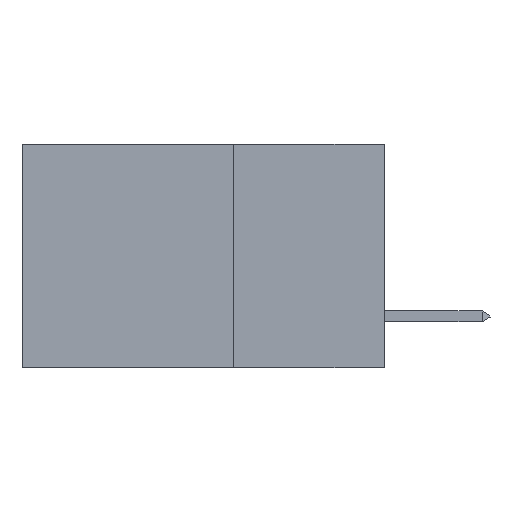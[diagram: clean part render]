
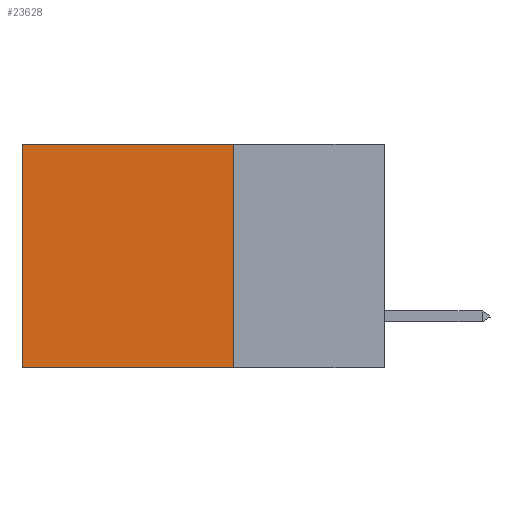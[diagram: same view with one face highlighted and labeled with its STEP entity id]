
A CAD part, left-side view. The second image highlights one B-rep face of the part: STEP entity #23628.
In plain terms, the highlighted planar face has unit normal (-1, 0, 0).
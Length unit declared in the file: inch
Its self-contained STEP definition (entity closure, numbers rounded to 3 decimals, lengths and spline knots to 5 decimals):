
#699 = FACE_OUTER_BOUND ( 'NONE', #1510, .T. ) ;
#1510 = EDGE_LOOP ( 'NONE', ( #21617, #4428, #1871, #13082 ) ) ;
#1652 = VECTOR ( 'NONE', #9317, 39.37008 ) ;
#1871 = ORIENTED_EDGE ( 'NONE', *, *, #20863, .F. ) ;
#3248 = CARTESIAN_POINT ( 'NONE',  ( 0.2875, 0.6, 0. ) ) ;
#3627 = VERTEX_POINT ( 'NONE', #20398 ) ;
#4079 = CARTESIAN_POINT ( 'NONE',  ( 0.2875, 0.25, -0.37 ) ) ;
#4428 = ORIENTED_EDGE ( 'NONE', *, *, #23830, .F. ) ;
#5561 = DIRECTION ( 'NONE',  ( 0., 0., -1. ) ) ;
#5659 = PLANE ( 'NONE',  #22956 ) ;
#5740 = VERTEX_POINT ( 'NONE', #3248 ) ;
#7494 = VECTOR ( 'NONE', #15050, 39.37008 ) ;
#7834 = CARTESIAN_POINT ( 'NONE',  ( 0.2875, 0.6, -0.37 ) ) ;
#8521 = EDGE_CURVE ( 'NONE', #21732, #5740, #12229, .T. ) ;
#8825 = VERTEX_POINT ( 'NONE', #7834 ) ;
#9296 = CARTESIAN_POINT ( 'NONE',  ( 0.2875, 0.25, 0. ) ) ;
#9317 = DIRECTION ( 'NONE',  ( 0., 1., 0. ) ) ;
#10477 = CARTESIAN_POINT ( 'NONE',  ( 0.2875, 0.6, 0. ) ) ;
#11054 = EDGE_CURVE ( 'NONE', #5740, #8825, #20104, .T. ) ;
#12229 = LINE ( 'NONE', #17716, #1652 ) ;
#13082 = ORIENTED_EDGE ( 'NONE', *, *, #8521, .T. ) ;
#15039 = VECTOR ( 'NONE', #23583, 39.37008 ) ;
#15050 = DIRECTION ( 'NONE',  ( 0., 1., 0. ) ) ;
#15095 = DIRECTION ( 'NONE',  ( 0., 0., -1. ) ) ;
#15701 = LINE ( 'NONE', #4079, #7494 ) ;
#15866 = LINE ( 'NONE', #9296, #18580 ) ;
#17716 = CARTESIAN_POINT ( 'NONE',  ( 0.2875, 0.25, 0. ) ) ;
#18580 = VECTOR ( 'NONE', #5561, 39.37008 ) ;
#18710 = DIRECTION ( 'NONE',  ( 1., 0., 0. ) ) ;
#18781 = CARTESIAN_POINT ( 'NONE',  ( 0.2875, 0.25, 0. ) ) ;
#20104 = LINE ( 'NONE', #10477, #15039 ) ;
#20398 = CARTESIAN_POINT ( 'NONE',  ( 0.2875, 0.25, -0.37 ) ) ;
#20863 = EDGE_CURVE ( 'NONE', #21732, #3627, #15866, .T. ) ;
#21617 = ORIENTED_EDGE ( 'NONE', *, *, #11054, .T. ) ;
#21732 = VERTEX_POINT ( 'NONE', #24199 ) ;
#22956 = AXIS2_PLACEMENT_3D ( 'NONE', #18781, #18710, #15095 ) ;
#23583 = DIRECTION ( 'NONE',  ( 0., 0., -1. ) ) ;
#23628 = ADVANCED_FACE ( 'NONE', ( #699 ), #5659, .F. ) ;
#23830 = EDGE_CURVE ( 'NONE', #3627, #8825, #15701, .T. ) ;
#24199 = CARTESIAN_POINT ( 'NONE',  ( 0.2875, 0.25, 0. ) ) ;
